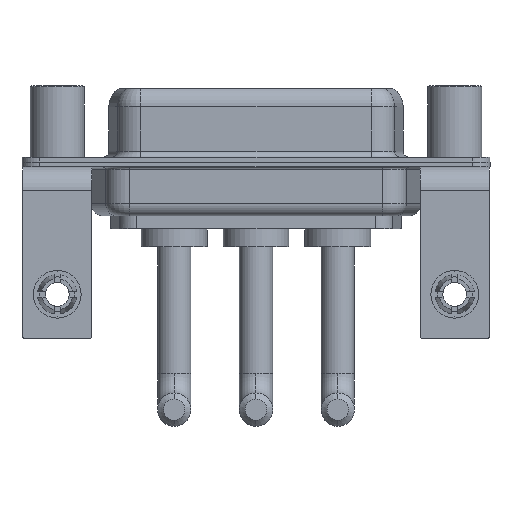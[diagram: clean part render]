
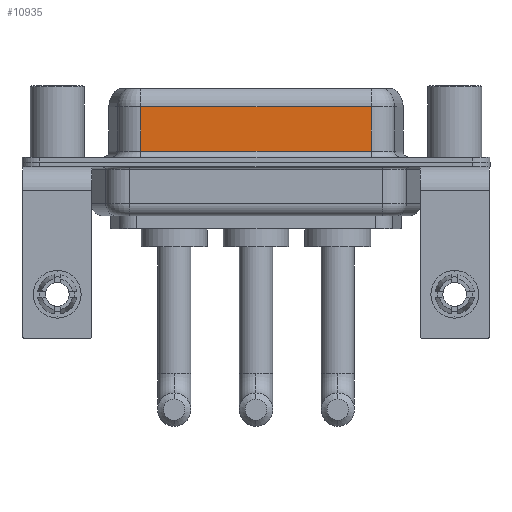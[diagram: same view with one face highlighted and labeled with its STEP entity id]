
A CAD part, front view. The second image highlights one B-rep face of the part: STEP entity #10935.
In plain terms, the highlighted planar face has unit normal (0, -1, 0).
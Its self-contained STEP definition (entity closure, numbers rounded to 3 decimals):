
#167 = LINE ( 'NONE', #7577, #8574 ) ;
#284 = EDGE_LOOP ( 'NONE', ( #1722, #2243, #14960, #3860 ) ) ;
#429 = CARTESIAN_POINT ( 'NONE',  ( 7.013, -3.95, 0.9 ) ) ;
#1437 = PLANE ( 'NONE',  #4374 ) ;
#1541 = VERTEX_POINT ( 'NONE', #12075 ) ;
#1670 = DIRECTION ( 'NONE',  ( -1., 0., 0. ) ) ;
#1722 = ORIENTED_EDGE ( 'NONE', *, *, #11702, .F. ) ;
#2243 = ORIENTED_EDGE ( 'NONE', *, *, #14474, .T. ) ;
#2938 = VERTEX_POINT ( 'NONE', #3148 ) ;
#2967 = EDGE_CURVE ( 'NONE', #12435, #2938, #11748, .T. ) ;
#3148 = CARTESIAN_POINT ( 'NONE',  ( 26.287, -3.95, 0.9 ) ) ;
#3645 = DIRECTION ( 'NONE',  ( 0., 0., -1. ) ) ;
#3715 = DIRECTION ( 'NONE',  ( 0., 1., 0. ) ) ;
#3786 = FACE_OUTER_BOUND ( 'NONE', #284, .T. ) ;
#3860 = ORIENTED_EDGE ( 'NONE', *, *, #2967, .T. ) ;
#3863 = CARTESIAN_POINT ( 'NONE',  ( 26.287, -3.95, 6.4 ) ) ;
#4100 = CARTESIAN_POINT ( 'NONE',  ( 26.287, -3.95, 4.65 ) ) ;
#4374 = AXIS2_PLACEMENT_3D ( 'NONE', #3863, #3715, #8771 ) ;
#5533 = DIRECTION ( 'NONE',  ( 0., 0., -1. ) ) ;
#5711 = DIRECTION ( 'NONE',  ( 1., 0., 0. ) ) ;
#6215 = VECTOR ( 'NONE', #1670, 1000. ) ;
#7052 = CARTESIAN_POINT ( 'NONE',  ( 26.287, -3.95, 6.4 ) ) ;
#7577 = CARTESIAN_POINT ( 'NONE',  ( 7.013, -3.95, 6.4 ) ) ;
#8125 = VERTEX_POINT ( 'NONE', #9102 ) ;
#8574 = VECTOR ( 'NONE', #3645, 1000. ) ;
#8771 = DIRECTION ( 'NONE',  ( 0., 0., 1. ) ) ;
#9102 = CARTESIAN_POINT ( 'NONE',  ( 26.287, -3.95, 4.65 ) ) ;
#10601 = EDGE_CURVE ( 'NONE', #1541, #12435, #167, .T. ) ;
#10935 = ADVANCED_FACE ( 'NONE', ( #3786 ), #1437, .F. ) ;
#11582 = CARTESIAN_POINT ( 'NONE',  ( 26.287, -3.95, 0.9 ) ) ;
#11702 = EDGE_CURVE ( 'NONE', #8125, #2938, #15407, .T. ) ;
#11748 = LINE ( 'NONE', #11582, #13873 ) ;
#12075 = CARTESIAN_POINT ( 'NONE',  ( 7.013, -3.95, 4.65 ) ) ;
#12435 = VERTEX_POINT ( 'NONE', #429 ) ;
#13080 = VECTOR ( 'NONE', #5533, 1000. ) ;
#13873 = VECTOR ( 'NONE', #5711, 1000. ) ;
#14474 = EDGE_CURVE ( 'NONE', #8125, #1541, #15108, .T. ) ;
#14960 = ORIENTED_EDGE ( 'NONE', *, *, #10601, .T. ) ;
#15108 = LINE ( 'NONE', #4100, #6215 ) ;
#15407 = LINE ( 'NONE', #7052, #13080 ) ;
